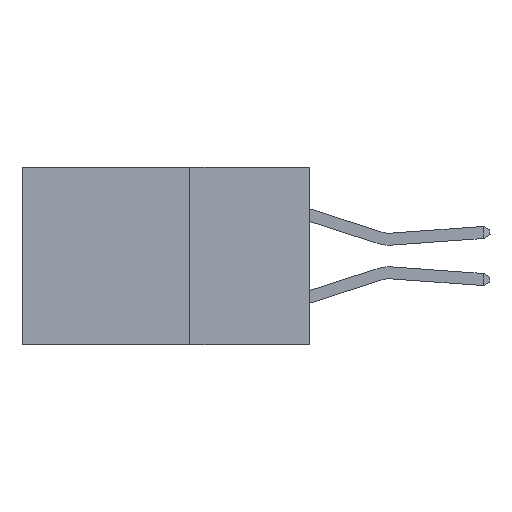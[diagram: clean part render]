
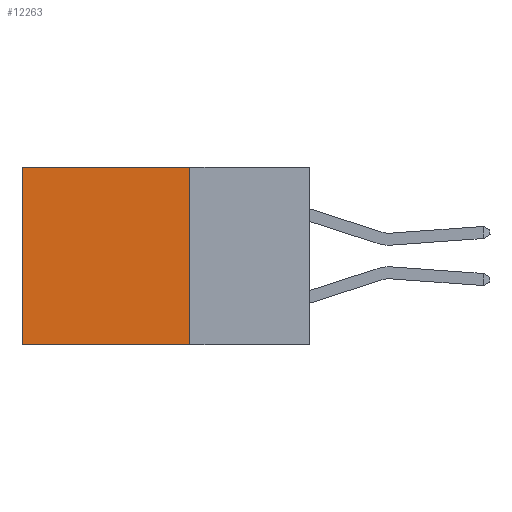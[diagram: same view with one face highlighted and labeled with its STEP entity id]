
A CAD part, left-side view. The second image highlights one B-rep face of the part: STEP entity #12263.
In plain terms, the highlighted planar face has unit normal (-1, 0, 0).
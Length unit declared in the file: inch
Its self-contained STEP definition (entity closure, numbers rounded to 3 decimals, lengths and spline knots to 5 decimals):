
#518 = VECTOR ( 'NONE', #10780, 39.37008 ) ;
#2502 = CARTESIAN_POINT ( 'NONE',  ( 0.2615, 0.25, -0.37 ) ) ;
#2840 = VERTEX_POINT ( 'NONE', #12794 ) ;
#2972 = EDGE_LOOP ( 'NONE', ( #4577, #7740, #14038, #14694 ) ) ;
#3316 = CARTESIAN_POINT ( 'NONE',  ( 0.2615, 0.25, -0.37 ) ) ;
#3615 = PLANE ( 'NONE',  #5869 ) ;
#4027 = DIRECTION ( 'NONE',  ( 0., 1., 0. ) ) ;
#4577 = ORIENTED_EDGE ( 'NONE', *, *, #9776, .T. ) ;
#5869 = AXIS2_PLACEMENT_3D ( 'NONE', #2502, #11471, #14022 ) ;
#6769 = LINE ( 'NONE', #13494, #518 ) ;
#7017 = CARTESIAN_POINT ( 'NONE',  ( 0.2615, 0.25, 0. ) ) ;
#7122 = VERTEX_POINT ( 'NONE', #11753 ) ;
#7740 = ORIENTED_EDGE ( 'NONE', *, *, #13756, .F. ) ;
#8261 = VERTEX_POINT ( 'NONE', #3316 ) ;
#8765 = DIRECTION ( 'NONE',  ( 0., 0., -1. ) ) ;
#9576 = CARTESIAN_POINT ( 'NONE',  ( 0.2615, 0.25, -0.37 ) ) ;
#9616 = LINE ( 'NONE', #16185, #11074 ) ;
#9618 = VECTOR ( 'NONE', #8765, 39.37008 ) ;
#9776 = EDGE_CURVE ( 'NONE', #2840, #7122, #11340, .T. ) ;
#10307 = CARTESIAN_POINT ( 'NONE',  ( 0.2615, 0.6, -0.37 ) ) ;
#10777 = LINE ( 'NONE', #9576, #16519 ) ;
#10780 = DIRECTION ( 'NONE',  ( 0., 0., -1. ) ) ;
#11074 = VECTOR ( 'NONE', #13615, 39.37008 ) ;
#11340 = LINE ( 'NONE', #10307, #9618 ) ;
#11471 = DIRECTION ( 'NONE',  ( 1., 0., 0. ) ) ;
#11753 = CARTESIAN_POINT ( 'NONE',  ( 0.2615, 0.6, -0.37 ) ) ;
#12263 = ADVANCED_FACE ( 'NONE', ( #13936 ), #3615, .F. ) ;
#12794 = CARTESIAN_POINT ( 'NONE',  ( 0.2615, 0.6, 0. ) ) ;
#13375 = EDGE_CURVE ( 'NONE', #16124, #2840, #9616, .T. ) ;
#13494 = CARTESIAN_POINT ( 'NONE',  ( 0.2615, 0.25, -0.37 ) ) ;
#13615 = DIRECTION ( 'NONE',  ( 0., 1., 0. ) ) ;
#13756 = EDGE_CURVE ( 'NONE', #8261, #7122, #10777, .T. ) ;
#13936 = FACE_OUTER_BOUND ( 'NONE', #2972, .T. ) ;
#14022 = DIRECTION ( 'NONE',  ( 0., 0., -1. ) ) ;
#14038 = ORIENTED_EDGE ( 'NONE', *, *, #16182, .F. ) ;
#14694 = ORIENTED_EDGE ( 'NONE', *, *, #13375, .T. ) ;
#16124 = VERTEX_POINT ( 'NONE', #7017 ) ;
#16182 = EDGE_CURVE ( 'NONE', #16124, #8261, #6769, .T. ) ;
#16185 = CARTESIAN_POINT ( 'NONE',  ( 0.2615, 0.25, 0. ) ) ;
#16519 = VECTOR ( 'NONE', #4027, 39.37008 ) ;
